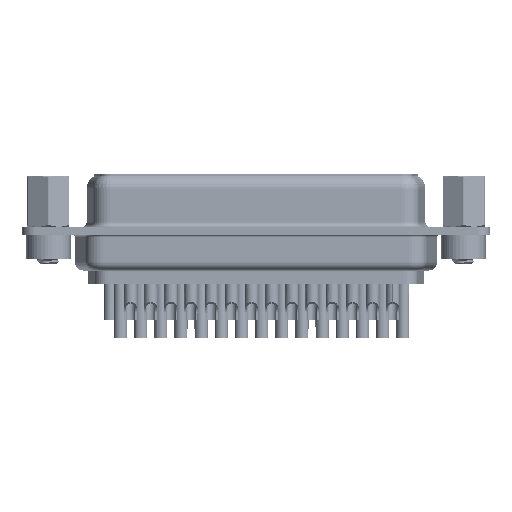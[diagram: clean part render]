
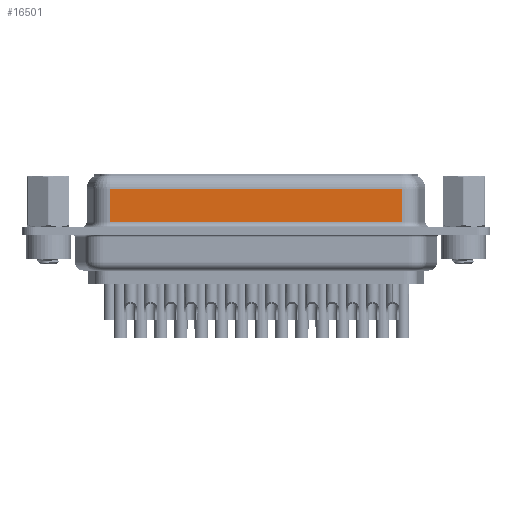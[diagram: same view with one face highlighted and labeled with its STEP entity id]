
A CAD part, front view. The second image highlights one B-rep face of the part: STEP entity #16501.
In plain terms, the highlighted planar face has unit normal (0, -1, 0).
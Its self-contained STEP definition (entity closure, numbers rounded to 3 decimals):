
#528 = CARTESIAN_POINT ( 'NONE',  ( 40.032, -3.95, 4.7 ) ) ;
#1399 = ORIENTED_EDGE ( 'NONE', *, *, #19870, .T. ) ;
#3170 = PLANE ( 'NONE',  #30958 ) ;
#3239 = LINE ( 'NONE', #15896, #6965 ) ;
#4930 = CARTESIAN_POINT ( 'NONE',  ( 40.032, -3.95, 4.7 ) ) ;
#5201 = CARTESIAN_POINT ( 'NONE',  ( 7.008, -3.95, 0.95 ) ) ;
#6965 = VECTOR ( 'NONE', #16094, 1000. ) ;
#8110 = VERTEX_POINT ( 'NONE', #528 ) ;
#8142 = CARTESIAN_POINT ( 'NONE',  ( 7.008, -3.95, 4.7 ) ) ;
#9003 = FACE_OUTER_BOUND ( 'NONE', #28767, .T. ) ;
#10012 = ORIENTED_EDGE ( 'NONE', *, *, #39957, .F. ) ;
#11429 = ORIENTED_EDGE ( 'NONE', *, *, #30316, .T. ) ;
#11941 = VERTEX_POINT ( 'NONE', #33437 ) ;
#13188 = CARTESIAN_POINT ( 'NONE',  ( 7.008, -3.95, 6.45 ) ) ;
#15828 = CARTESIAN_POINT ( 'NONE',  ( 40.032, -3.95, 6.45 ) ) ;
#15896 = CARTESIAN_POINT ( 'NONE',  ( 40.032, -3.95, 0.95 ) ) ;
#16094 = DIRECTION ( 'NONE',  ( 1., 0., 0. ) ) ;
#16501 = ADVANCED_FACE ( 'NONE', ( #9003 ), #3170, .F. ) ;
#16997 = DIRECTION ( 'NONE',  ( -1., 0., 0. ) ) ;
#19870 = EDGE_CURVE ( 'NONE', #30816, #29996, #22518, .T. ) ;
#20330 = EDGE_CURVE ( 'NONE', #29996, #11941, #3239, .T. ) ;
#20727 = LINE ( 'NONE', #4930, #29994 ) ;
#21182 = VECTOR ( 'NONE', #36298, 1000. ) ;
#22518 = LINE ( 'NONE', #13188, #39355 ) ;
#24753 = DIRECTION ( 'NONE',  ( 0., 0., 1. ) ) ;
#25482 = ORIENTED_EDGE ( 'NONE', *, *, #20330, .T. ) ;
#26453 = DIRECTION ( 'NONE',  ( 0., 0., -1. ) ) ;
#28767 = EDGE_LOOP ( 'NONE', ( #10012, #11429, #1399, #25482 ) ) ;
#29994 = VECTOR ( 'NONE', #16997, 1000. ) ;
#29996 = VERTEX_POINT ( 'NONE', #5201 ) ;
#30316 = EDGE_CURVE ( 'NONE', #8110, #30816, #20727, .T. ) ;
#30816 = VERTEX_POINT ( 'NONE', #8142 ) ;
#30958 = AXIS2_PLACEMENT_3D ( 'NONE', #15828, #37587, #24753 ) ;
#32591 = LINE ( 'NONE', #36102, #21182 ) ;
#33437 = CARTESIAN_POINT ( 'NONE',  ( 40.032, -3.95, 0.95 ) ) ;
#36102 = CARTESIAN_POINT ( 'NONE',  ( 40.032, -3.95, 6.45 ) ) ;
#36298 = DIRECTION ( 'NONE',  ( 0., 0., -1. ) ) ;
#37587 = DIRECTION ( 'NONE',  ( 0., 1., 0. ) ) ;
#39355 = VECTOR ( 'NONE', #26453, 1000. ) ;
#39957 = EDGE_CURVE ( 'NONE', #8110, #11941, #32591, .T. ) ;
